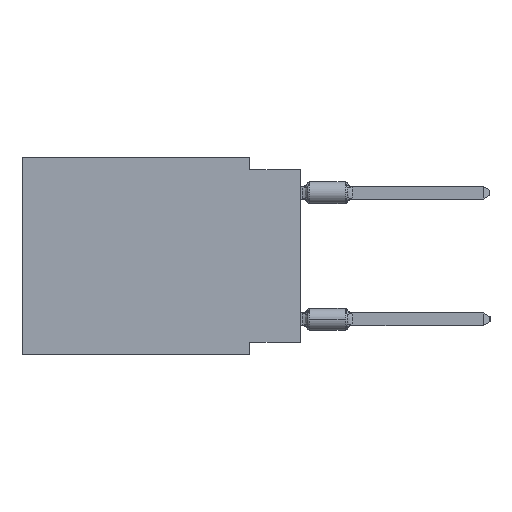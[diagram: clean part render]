
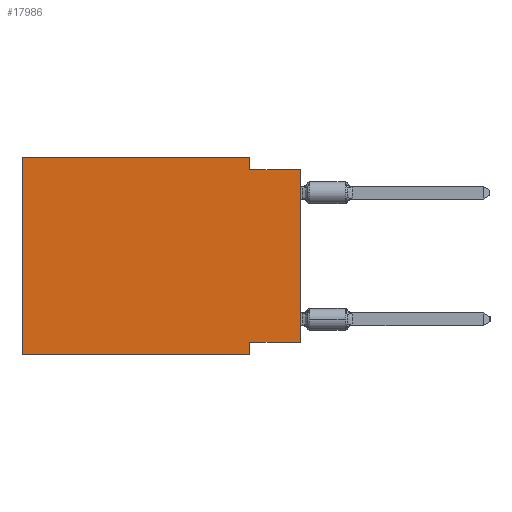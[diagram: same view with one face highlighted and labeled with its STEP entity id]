
A CAD part, left-side view. The second image highlights one B-rep face of the part: STEP entity #17986.
In plain terms, the highlighted planar face has unit normal (-1, 0, 0).
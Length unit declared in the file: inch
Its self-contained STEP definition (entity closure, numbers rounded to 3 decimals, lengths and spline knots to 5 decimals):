
#197 = DIRECTION ( 'NONE',  ( 0., 0., -1. ) ) ;
#755 = VERTEX_POINT ( 'NONE', #19367 ) ;
#2036 = CARTESIAN_POINT ( 'NONE',  ( 0., 0.55, -0.39 ) ) ;
#2053 = VECTOR ( 'NONE', #197, 39.37008 ) ;
#2175 = EDGE_LOOP ( 'NONE', ( #11594, #8279, #9665, #18827, #7991, #13700, #27811, #21220 ) ) ;
#2345 = LINE ( 'NONE', #19861, #2053 ) ;
#3583 = CARTESIAN_POINT ( 'NONE',  ( 0., 0., -0.025 ) ) ;
#4983 = VERTEX_POINT ( 'NONE', #2036 ) ;
#5200 = VECTOR ( 'NONE', #7951, 39.37008 ) ;
#5413 = CARTESIAN_POINT ( 'NONE',  ( 0., 0.55, 0. ) ) ;
#5415 = CARTESIAN_POINT ( 'NONE',  ( 0., 0.1, 0. ) ) ;
#6477 = VECTOR ( 'NONE', #13928, 39.37008 ) ;
#6482 = DIRECTION ( 'NONE',  ( 0., 0., 1. ) ) ;
#7038 = LINE ( 'NONE', #26571, #25339 ) ;
#7064 = CARTESIAN_POINT ( 'NONE',  ( 0., 0.1, -0.365 ) ) ;
#7951 = DIRECTION ( 'NONE',  ( 0., 1., 0. ) ) ;
#7991 = ORIENTED_EDGE ( 'NONE', *, *, #24293, .F. ) ;
#8114 = LINE ( 'NONE', #5413, #22607 ) ;
#8279 = ORIENTED_EDGE ( 'NONE', *, *, #25185, .F. ) ;
#8635 = LINE ( 'NONE', #13109, #23859 ) ;
#9608 = LINE ( 'NONE', #18239, #6477 ) ;
#9665 = ORIENTED_EDGE ( 'NONE', *, *, #19125, .F. ) ;
#9750 = CARTESIAN_POINT ( 'NONE',  ( 0., 0.55, -0.39 ) ) ;
#11114 = VERTEX_POINT ( 'NONE', #7064 ) ;
#11117 = VECTOR ( 'NONE', #16233, 39.37008 ) ;
#11276 = CARTESIAN_POINT ( 'NONE',  ( 0., 0.55, 0. ) ) ;
#11594 = ORIENTED_EDGE ( 'NONE', *, *, #17343, .T. ) ;
#11667 = EDGE_CURVE ( 'NONE', #4983, #14418, #20392, .T. ) ;
#12202 = EDGE_CURVE ( 'NONE', #21321, #11114, #23179, .T. ) ;
#12486 = DIRECTION ( 'NONE',  ( 0., 0., -1. ) ) ;
#13109 = CARTESIAN_POINT ( 'NONE',  ( 0., 0., 0. ) ) ;
#13615 = EDGE_CURVE ( 'NONE', #11114, #14418, #2345, .T. ) ;
#13700 = ORIENTED_EDGE ( 'NONE', *, *, #11667, .T. ) ;
#13915 = VECTOR ( 'NONE', #20948, 39.37008 ) ;
#13928 = DIRECTION ( 'NONE',  ( 0., 0., -1. ) ) ;
#14418 = VERTEX_POINT ( 'NONE', #20346 ) ;
#16233 = DIRECTION ( 'NONE',  ( 0., -1., 0. ) ) ;
#16652 = CARTESIAN_POINT ( 'NONE',  ( 0., 0.55, 0. ) ) ;
#16753 = VERTEX_POINT ( 'NONE', #5415 ) ;
#16889 = CARTESIAN_POINT ( 'NONE',  ( 0., 0., -0.365 ) ) ;
#17343 = EDGE_CURVE ( 'NONE', #21321, #24313, #8635, .T. ) ;
#17986 = ADVANCED_FACE ( 'NONE', ( #27434 ), #22954, .F. ) ;
#18239 = CARTESIAN_POINT ( 'NONE',  ( 0., 0.1, 0. ) ) ;
#18527 = DIRECTION ( 'NONE',  ( 1., 0., 0. ) ) ;
#18623 = CARTESIAN_POINT ( 'NONE',  ( 0., 0., -0.025 ) ) ;
#18827 = ORIENTED_EDGE ( 'NONE', *, *, #22428, .F. ) ;
#19125 = EDGE_CURVE ( 'NONE', #16753, #755, #9608, .T. ) ;
#19367 = CARTESIAN_POINT ( 'NONE',  ( 0., 0.1, -0.025 ) ) ;
#19861 = CARTESIAN_POINT ( 'NONE',  ( 0., 0.1, -0.39 ) ) ;
#20346 = CARTESIAN_POINT ( 'NONE',  ( 0., 0.1, -0.39 ) ) ;
#20392 = LINE ( 'NONE', #9750, #11117 ) ;
#20948 = DIRECTION ( 'NONE',  ( 0., -1., 0. ) ) ;
#21220 = ORIENTED_EDGE ( 'NONE', *, *, #12202, .F. ) ;
#21321 = VERTEX_POINT ( 'NONE', #16889 ) ;
#22428 = EDGE_CURVE ( 'NONE', #22586, #16753, #7038, .T. ) ;
#22586 = VERTEX_POINT ( 'NONE', #11276 ) ;
#22607 = VECTOR ( 'NONE', #25084, 39.37008 ) ;
#22954 = PLANE ( 'NONE',  #27109 ) ;
#23179 = LINE ( 'NONE', #27645, #5200 ) ;
#23659 = LINE ( 'NONE', #3583, #13915 ) ;
#23859 = VECTOR ( 'NONE', #6482, 39.37008 ) ;
#24293 = EDGE_CURVE ( 'NONE', #4983, #22586, #8114, .T. ) ;
#24313 = VERTEX_POINT ( 'NONE', #18623 ) ;
#25084 = DIRECTION ( 'NONE',  ( 0., 0., 1. ) ) ;
#25185 = EDGE_CURVE ( 'NONE', #755, #24313, #23659, .T. ) ;
#25339 = VECTOR ( 'NONE', #26879, 39.37008 ) ;
#26571 = CARTESIAN_POINT ( 'NONE',  ( 0., 0.55, 0. ) ) ;
#26879 = DIRECTION ( 'NONE',  ( 0., -1., 0. ) ) ;
#27109 = AXIS2_PLACEMENT_3D ( 'NONE', #16652, #18527, #12486 ) ;
#27434 = FACE_OUTER_BOUND ( 'NONE', #2175, .T. ) ;
#27645 = CARTESIAN_POINT ( 'NONE',  ( 0., 0., -0.365 ) ) ;
#27811 = ORIENTED_EDGE ( 'NONE', *, *, #13615, .F. ) ;
